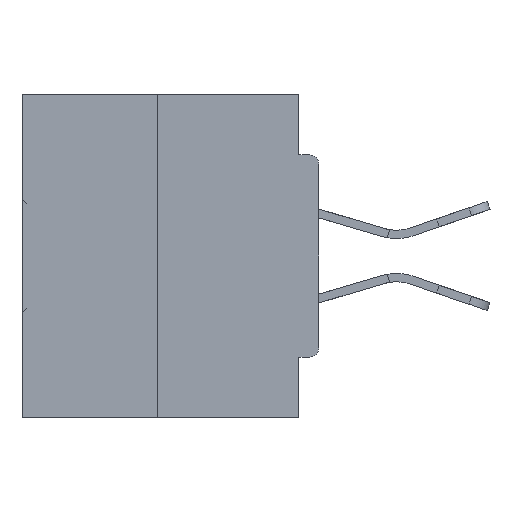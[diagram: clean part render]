
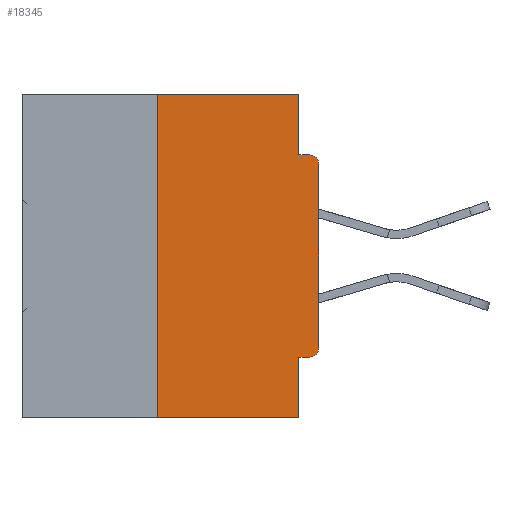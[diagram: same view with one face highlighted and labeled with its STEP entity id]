
A CAD part, left-side view. The second image highlights one B-rep face of the part: STEP entity #18345.
In plain terms, the highlighted planar face has unit normal (-1, 0, 0).
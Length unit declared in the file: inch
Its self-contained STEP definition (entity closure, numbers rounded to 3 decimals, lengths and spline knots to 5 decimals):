
#158 = DIRECTION ( 'NONE',  ( 0., 0., -1. ) ) ;
#372 = AXIS2_PLACEMENT_3D ( 'NONE', #40883, #4702, #33930 ) ;
#403 = EDGE_CURVE ( 'NONE', #20466, #6804, #27769, .T. ) ;
#832 = EDGE_CURVE ( 'NONE', #2832, #21278, #33980, .T. ) ;
#1472 = CARTESIAN_POINT ( 'NONE',  ( 0., 0., -0.1085 ) ) ;
#1553 = EDGE_CURVE ( 'NONE', #31291, #6592, #5288, .T. ) ;
#2203 = DIRECTION ( 'NONE',  ( 0., 0., -1. ) ) ;
#2832 = VERTEX_POINT ( 'NONE', #21368 ) ;
#3434 = EDGE_CURVE ( 'NONE', #2832, #15079, #7424, .T. ) ;
#4434 = VECTOR ( 'NONE', #4798, 39.37008 ) ;
#4620 = ORIENTED_EDGE ( 'NONE', *, *, #43084, .T. ) ;
#4702 = DIRECTION ( 'NONE',  ( -1., 0., 0. ) ) ;
#4798 = DIRECTION ( 'NONE',  ( 0., -1., 0. ) ) ;
#5259 = VERTEX_POINT ( 'NONE', #13146 ) ;
#5288 = LINE ( 'NONE', #28647, #15591 ) ;
#5419 = ORIENTED_EDGE ( 'NONE', *, *, #17036, .F. ) ;
#6474 = FACE_OUTER_BOUND ( 'NONE', #12807, .T. ) ;
#6491 = CARTESIAN_POINT ( 'NONE',  ( 0., 0.031, 0. ) ) ;
#6592 = VERTEX_POINT ( 'NONE', #19733 ) ;
#6804 = VERTEX_POINT ( 'NONE', #47169 ) ;
#7424 = CIRCLE ( 'NONE', #372, 0.015 ) ;
#7663 = ORIENTED_EDGE ( 'NONE', *, *, #15903, .T. ) ;
#7996 = EDGE_CURVE ( 'NONE', #5259, #20466, #33615, .T. ) ;
#8597 = DIRECTION ( 'NONE',  ( 0., 0., -1. ) ) ;
#10420 = VECTOR ( 'NONE', #8597, 39.37008 ) ;
#10552 = VECTOR ( 'NONE', #17044, 39.37008 ) ;
#11974 = EDGE_CURVE ( 'NONE', #21278, #6592, #20102, .T. ) ;
#12079 = ORIENTED_EDGE ( 'NONE', *, *, #832, .F. ) ;
#12268 = VERTEX_POINT ( 'NONE', #1472 ) ;
#12543 = LINE ( 'NONE', #41550, #40475 ) ;
#12807 = EDGE_LOOP ( 'NONE', ( #43387, #29375, #19503, #35102, #12079, #31718, #4620, #7663, #5419, #44937 ) ) ;
#13146 = CARTESIAN_POINT ( 'NONE',  ( 0., 0.25, 0. ) ) ;
#14002 = DIRECTION ( 'NONE',  ( 0., 0., -1. ) ) ;
#15079 = VERTEX_POINT ( 'NONE', #18613 ) ;
#15591 = VECTOR ( 'NONE', #46972, 39.37008 ) ;
#15903 = EDGE_CURVE ( 'NONE', #12268, #22472, #33579, .T. ) ;
#17036 = EDGE_CURVE ( 'NONE', #6804, #22472, #19701, .T. ) ;
#17044 = DIRECTION ( 'NONE',  ( 0., 1., 0. ) ) ;
#17735 = DIRECTION ( 'NONE',  ( 0., 0., 1. ) ) ;
#18345 = ADVANCED_FACE ( 'NONE', ( #6474 ), #45086, .F. ) ;
#18613 = CARTESIAN_POINT ( 'NONE',  ( 0., 0., -0.3915 ) ) ;
#18828 = CARTESIAN_POINT ( 'NONE',  ( 0., 0.015, -0.0935 ) ) ;
#19503 = ORIENTED_EDGE ( 'NONE', *, *, #1553, .T. ) ;
#19701 = LINE ( 'NONE', #47114, #32317 ) ;
#19733 = CARTESIAN_POINT ( 'NONE',  ( 0., 0.031, -0.5 ) ) ;
#20102 = LINE ( 'NONE', #37635, #10420 ) ;
#20427 = VECTOR ( 'NONE', #17735, 39.37008 ) ;
#20466 = VERTEX_POINT ( 'NONE', #6491 ) ;
#20785 = CARTESIAN_POINT ( 'NONE',  ( 0., 0., 0. ) ) ;
#21278 = VERTEX_POINT ( 'NONE', #42366 ) ;
#21368 = CARTESIAN_POINT ( 'NONE',  ( 0., 0.015, -0.4065 ) ) ;
#21511 = DIRECTION ( 'NONE',  ( -1., 0., 0. ) ) ;
#22154 = EDGE_CURVE ( 'NONE', #31291, #5259, #12543, .T. ) ;
#22472 = VERTEX_POINT ( 'NONE', #18828 ) ;
#23441 = CARTESIAN_POINT ( 'NONE',  ( 0., 0.46, 0. ) ) ;
#24856 = CARTESIAN_POINT ( 'NONE',  ( 0., 0.25, -0.5 ) ) ;
#24893 = CARTESIAN_POINT ( 'NONE',  ( 0., 0.015, -0.1085 ) ) ;
#27100 = DIRECTION ( 'NONE',  ( 1., 0., 0. ) ) ;
#27160 = VECTOR ( 'NONE', #158, 39.37008 ) ;
#27769 = LINE ( 'NONE', #33677, #27160 ) ;
#28647 = CARTESIAN_POINT ( 'NONE',  ( 0., 0.46, -0.5 ) ) ;
#29375 = ORIENTED_EDGE ( 'NONE', *, *, #22154, .F. ) ;
#30778 = DIRECTION ( 'NONE',  ( 0., 0., 1. ) ) ;
#31291 = VERTEX_POINT ( 'NONE', #24856 ) ;
#31718 = ORIENTED_EDGE ( 'NONE', *, *, #3434, .T. ) ;
#32317 = VECTOR ( 'NONE', #43093, 39.37008 ) ;
#33579 = CIRCLE ( 'NONE', #40508, 0.015 ) ;
#33615 = LINE ( 'NONE', #44978, #4434 ) ;
#33677 = CARTESIAN_POINT ( 'NONE',  ( 0., 0.031, 0. ) ) ;
#33930 = DIRECTION ( 'NONE',  ( 0., 0., -1. ) ) ;
#33980 = LINE ( 'NONE', #39349, #10552 ) ;
#35102 = ORIENTED_EDGE ( 'NONE', *, *, #11974, .F. ) ;
#37635 = CARTESIAN_POINT ( 'NONE',  ( 0., 0.031, -0.5 ) ) ;
#39349 = CARTESIAN_POINT ( 'NONE',  ( 0., 0., -0.4065 ) ) ;
#40475 = VECTOR ( 'NONE', #30778, 39.37008 ) ;
#40508 = AXIS2_PLACEMENT_3D ( 'NONE', #24893, #21511, #14002 ) ;
#40883 = CARTESIAN_POINT ( 'NONE',  ( 0., 0.015, -0.3915 ) ) ;
#41550 = CARTESIAN_POINT ( 'NONE',  ( 0., 0.25, 0. ) ) ;
#42366 = CARTESIAN_POINT ( 'NONE',  ( 0., 0.031, -0.4065 ) ) ;
#43084 = EDGE_CURVE ( 'NONE', #15079, #12268, #45552, .T. ) ;
#43093 = DIRECTION ( 'NONE',  ( 0., -1., 0. ) ) ;
#43387 = ORIENTED_EDGE ( 'NONE', *, *, #7996, .F. ) ;
#44937 = ORIENTED_EDGE ( 'NONE', *, *, #403, .F. ) ;
#44978 = CARTESIAN_POINT ( 'NONE',  ( 0., 0.46, 0. ) ) ;
#45086 = PLANE ( 'NONE',  #47065 ) ;
#45552 = LINE ( 'NONE', #20785, #20427 ) ;
#46972 = DIRECTION ( 'NONE',  ( 0., -1., 0. ) ) ;
#47065 = AXIS2_PLACEMENT_3D ( 'NONE', #23441, #27100, #2203 ) ;
#47114 = CARTESIAN_POINT ( 'NONE',  ( 0., 0., -0.0935 ) ) ;
#47169 = CARTESIAN_POINT ( 'NONE',  ( 0., 0.031, -0.0935 ) ) ;
